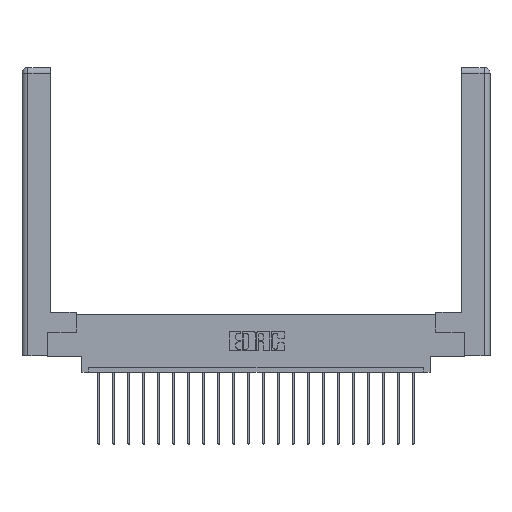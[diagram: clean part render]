
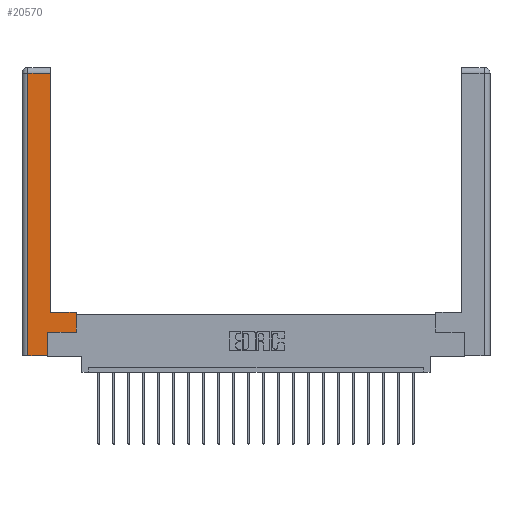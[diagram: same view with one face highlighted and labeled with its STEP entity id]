
A CAD part, top view. The second image highlights one B-rep face of the part: STEP entity #20570.
In plain terms, the highlighted planar face has unit normal (0, 0, 1).
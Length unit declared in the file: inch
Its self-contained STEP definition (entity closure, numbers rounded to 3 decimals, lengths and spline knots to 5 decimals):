
#1280 = CARTESIAN_POINT ( 'NONE',  ( 0.265, 0., 0. ) ) ;
#1411 = DIRECTION ( 'NONE',  ( 0., 1., 0. ) ) ;
#2059 = CARTESIAN_POINT ( 'NONE',  ( 0.295, 0.45, 0. ) ) ;
#2413 = CARTESIAN_POINT ( 'NONE',  ( 0., 0., 0. ) ) ;
#2496 = CARTESIAN_POINT ( 'NONE',  ( 0.565, 0.245, 0. ) ) ;
#3150 = EDGE_CURVE ( 'NONE', #8151, #16426, #13650, .T. ) ;
#3483 = ORIENTED_EDGE ( 'NONE', *, *, #12836, .T. ) ;
#3683 = VECTOR ( 'NONE', #19246, 39.37008 ) ;
#3866 = VECTOR ( 'NONE', #1411, 39.37008 ) ;
#4445 = VECTOR ( 'NONE', #14058, 39.37008 ) ;
#4499 = AXIS2_PLACEMENT_3D ( 'NONE', #2413, #14471, #16251 ) ;
#4617 = ORIENTED_EDGE ( 'NONE', *, *, #14829, .T. ) ;
#4633 = EDGE_CURVE ( 'NONE', #16426, #18194, #5448, .T. ) ;
#5157 = LINE ( 'NONE', #21479, #3866 ) ;
#5448 = LINE ( 'NONE', #9398, #20395 ) ;
#5702 = PLANE ( 'NONE',  #4499 ) ;
#5793 = CARTESIAN_POINT ( 'NONE',  ( 0.295, 2.94, 0. ) ) ;
#6112 = CARTESIAN_POINT ( 'NONE',  ( 0.295, 0.45, 0. ) ) ;
#6257 = LINE ( 'NONE', #7464, #3683 ) ;
#6265 = VERTEX_POINT ( 'NONE', #6112 ) ;
#7464 = CARTESIAN_POINT ( 'NONE',  ( 0.295, 3., 0. ) ) ;
#7671 = VERTEX_POINT ( 'NONE', #12683 ) ;
#8007 = VECTOR ( 'NONE', #12687, 39.37008 ) ;
#8151 = VERTEX_POINT ( 'NONE', #5793 ) ;
#8213 = CARTESIAN_POINT ( 'NONE',  ( 0.565, 0.45, 0. ) ) ;
#8829 = ORIENTED_EDGE ( 'NONE', *, *, #15503, .T. ) ;
#9218 = VECTOR ( 'NONE', #20194, 39.37008 ) ;
#9398 = CARTESIAN_POINT ( 'NONE',  ( 0.0615, 0., 0. ) ) ;
#10065 = VERTEX_POINT ( 'NONE', #14909 ) ;
#10592 = LINE ( 'NONE', #2496, #14195 ) ;
#10952 = DIRECTION ( 'NONE',  ( 1., 0., 0. ) ) ;
#11250 = FACE_OUTER_BOUND ( 'NONE', #20416, .T. ) ;
#12608 = CARTESIAN_POINT ( 'NONE',  ( 0.0615, 2.94, 0. ) ) ;
#12619 = ORIENTED_EDGE ( 'NONE', *, *, #3150, .T. ) ;
#12683 = CARTESIAN_POINT ( 'NONE',  ( 0.265, 0., 0. ) ) ;
#12687 = DIRECTION ( 'NONE',  ( 0., 1., 0. ) ) ;
#12836 = EDGE_CURVE ( 'NONE', #21020, #10065, #10592, .T. ) ;
#13650 = LINE ( 'NONE', #21649, #9218 ) ;
#13671 = ORIENTED_EDGE ( 'NONE', *, *, #4633, .T. ) ;
#13893 = ORIENTED_EDGE ( 'NONE', *, *, #14347, .T. ) ;
#13895 = VERTEX_POINT ( 'NONE', #8213 ) ;
#14058 = DIRECTION ( 'NONE',  ( -1., 0., 0. ) ) ;
#14195 = VECTOR ( 'NONE', #10952, 39.37008 ) ;
#14278 = LINE ( 'NONE', #19329, #8007 ) ;
#14347 = EDGE_CURVE ( 'NONE', #18194, #7671, #19056, .T. ) ;
#14471 = DIRECTION ( 'NONE',  ( 0., 0., -1. ) ) ;
#14829 = EDGE_CURVE ( 'NONE', #7671, #21020, #5157, .T. ) ;
#14909 = CARTESIAN_POINT ( 'NONE',  ( 0.565, 0.245, 0. ) ) ;
#15350 = CARTESIAN_POINT ( 'NONE',  ( 0.0615, 0., 0. ) ) ;
#15503 = EDGE_CURVE ( 'NONE', #10065, #13895, #14278, .T. ) ;
#16251 = DIRECTION ( 'NONE',  ( -1., 0., 0. ) ) ;
#16395 = DIRECTION ( 'NONE',  ( 1., 0., 0. ) ) ;
#16426 = VERTEX_POINT ( 'NONE', #12608 ) ;
#17504 = VECTOR ( 'NONE', #16395, 39.37008 ) ;
#17642 = ORIENTED_EDGE ( 'NONE', *, *, #18921, .T. ) ;
#17818 = ORIENTED_EDGE ( 'NONE', *, *, #18847, .T. ) ;
#18194 = VERTEX_POINT ( 'NONE', #15350 ) ;
#18780 = CARTESIAN_POINT ( 'NONE',  ( 0.265, 0.245, 0. ) ) ;
#18839 = LINE ( 'NONE', #2059, #4445 ) ;
#18847 = EDGE_CURVE ( 'NONE', #13895, #6265, #18839, .T. ) ;
#18921 = EDGE_CURVE ( 'NONE', #6265, #8151, #6257, .T. ) ;
#19056 = LINE ( 'NONE', #1280, #17504 ) ;
#19246 = DIRECTION ( 'NONE',  ( 0., 1., 0. ) ) ;
#19329 = CARTESIAN_POINT ( 'NONE',  ( 0.565, 0.45, 0. ) ) ;
#20194 = DIRECTION ( 'NONE',  ( -1., 0., 0. ) ) ;
#20395 = VECTOR ( 'NONE', #21087, 39.37008 ) ;
#20416 = EDGE_LOOP ( 'NONE', ( #17642, #12619, #13671, #13893, #4617, #3483, #8829, #17818 ) ) ;
#20570 = ADVANCED_FACE ( 'NONE', ( #11250 ), #5702, .F. ) ;
#21020 = VERTEX_POINT ( 'NONE', #18780 ) ;
#21087 = DIRECTION ( 'NONE',  ( 0., -1., 0. ) ) ;
#21479 = CARTESIAN_POINT ( 'NONE',  ( 0.265, 0.245, 0. ) ) ;
#21649 = CARTESIAN_POINT ( 'NONE',  ( 0.0615, 2.94, 0. ) ) ;
